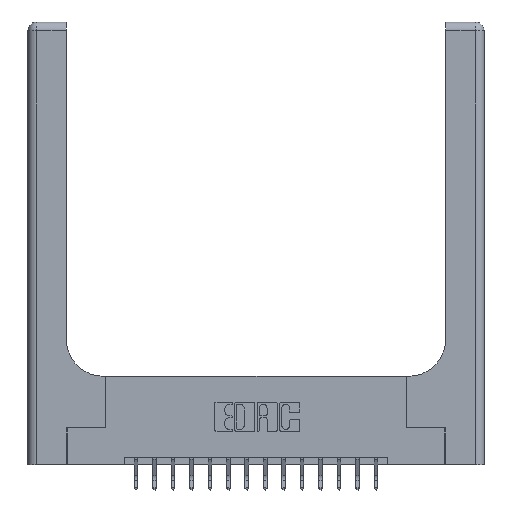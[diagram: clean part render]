
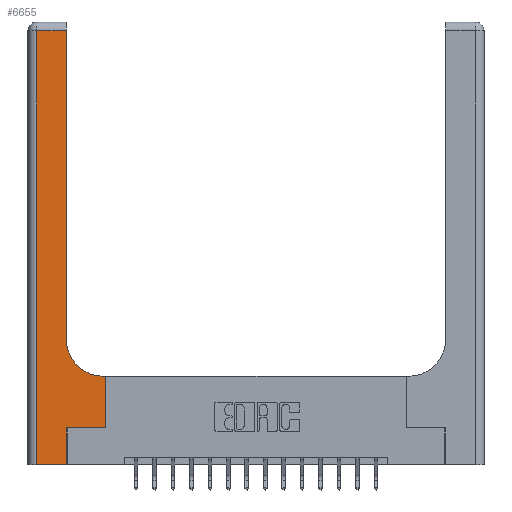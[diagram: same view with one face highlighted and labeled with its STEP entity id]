
A CAD part, top view. The second image highlights one B-rep face of the part: STEP entity #6655.
In plain terms, the highlighted planar face has unit normal (0, 0, 1).
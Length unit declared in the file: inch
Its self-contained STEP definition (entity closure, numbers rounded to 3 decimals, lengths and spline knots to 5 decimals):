
#21 = CARTESIAN_POINT ( 'NONE',  ( 0.265, 0.25, 0.37 ) ) ;
#148 = EDGE_CURVE ( 'NONE', #16364, #14837, #5709, .T. ) ;
#1210 = VECTOR ( 'NONE', #6075, 39.37008 ) ;
#1380 = CARTESIAN_POINT ( 'NONE',  ( 0.265, 0., 0.37 ) ) ;
#1383 = VERTEX_POINT ( 'NONE', #8633 ) ;
#1597 = EDGE_CURVE ( 'NONE', #13291, #3685, #11642, .T. ) ;
#2783 = DIRECTION ( 'NONE',  ( 0., 1., 0. ) ) ;
#3104 = DIRECTION ( 'NONE',  ( 1., 0., 0. ) ) ;
#3341 = DIRECTION ( 'NONE',  ( 0., -1., 0. ) ) ;
#3344 = DIRECTION ( 'NONE',  ( 0., 0., -1. ) ) ;
#3593 = CARTESIAN_POINT ( 'NONE',  ( 0.528, 0.25, 0.37 ) ) ;
#3625 = ORIENTED_EDGE ( 'NONE', *, *, #1597, .T. ) ;
#3685 = VERTEX_POINT ( 'NONE', #4628 ) ;
#3736 = EDGE_CURVE ( 'NONE', #1383, #4712, #17522, .T. ) ;
#4628 = CARTESIAN_POINT ( 'NONE',  ( 0.51, 0.6, 0.37 ) ) ;
#4673 = CARTESIAN_POINT ( 'NONE',  ( 0., 3., 0.37 ) ) ;
#4712 = VERTEX_POINT ( 'NONE', #1380 ) ;
#4831 = LINE ( 'NONE', #5018, #13030 ) ;
#5018 = CARTESIAN_POINT ( 'NONE',  ( 0.26, 3., 0.37 ) ) ;
#5105 = VERTEX_POINT ( 'NONE', #17674 ) ;
#5141 = CARTESIAN_POINT ( 'NONE',  ( 0.528, 0.25, 0.37 ) ) ;
#5709 = LINE ( 'NONE', #21, #10690 ) ;
#5746 = VECTOR ( 'NONE', #2783, 39.37008 ) ;
#5794 = DIRECTION ( 'NONE',  ( 1., 0., 0. ) ) ;
#6075 = DIRECTION ( 'NONE',  ( -1., 0., 0. ) ) ;
#6405 = CARTESIAN_POINT ( 'NONE',  ( 0.51, 0.85, 0.37 ) ) ;
#6655 = ADVANCED_FACE ( 'NONE', ( #17668 ), #13672, .F. ) ;
#6920 = ORIENTED_EDGE ( 'NONE', *, *, #13855, .T. ) ;
#6941 = ORIENTED_EDGE ( 'NONE', *, *, #12118, .T. ) ;
#7020 = EDGE_CURVE ( 'NONE', #5105, #18494, #11986, .T. ) ;
#7134 = EDGE_CURVE ( 'NONE', #7585, #5105, #4831, .T. ) ;
#7201 = ORIENTED_EDGE ( 'NONE', *, *, #7134, .T. ) ;
#7532 = CARTESIAN_POINT ( 'NONE',  ( 0.26, 0.6, 0.37 ) ) ;
#7585 = VERTEX_POINT ( 'NONE', #15391 ) ;
#8453 = EDGE_CURVE ( 'NONE', #4712, #16364, #10010, .T. ) ;
#8633 = CARTESIAN_POINT ( 'NONE',  ( 0.06, 0., 0.37 ) ) ;
#8714 = VECTOR ( 'NONE', #3104, 39.37008 ) ;
#9379 = DIRECTION ( 'NONE',  ( 0., 1., 0. ) ) ;
#10010 = LINE ( 'NONE', #15774, #5746 ) ;
#10304 = EDGE_CURVE ( 'NONE', #18494, #1383, #10725, .T. ) ;
#10545 = DIRECTION ( 'NONE',  ( -1., 0., 0. ) ) ;
#10690 = VECTOR ( 'NONE', #5794, 39.37008 ) ;
#10709 = DIRECTION ( 'NONE',  ( 1., 0., 0. ) ) ;
#10725 = LINE ( 'NONE', #13668, #15811 ) ;
#11341 = VECTOR ( 'NONE', #13161, 39.37008 ) ;
#11504 = AXIS2_PLACEMENT_3D ( 'NONE', #4673, #3344, #10545 ) ;
#11642 = LINE ( 'NONE', #7532, #11341 ) ;
#11924 = ORIENTED_EDGE ( 'NONE', *, *, #7020, .T. ) ;
#11986 = LINE ( 'NONE', #13596, #1210 ) ;
#12118 = EDGE_CURVE ( 'NONE', #3685, #7585, #17019, .T. ) ;
#12216 = DIRECTION ( 'NONE',  ( 0., 1., 0. ) ) ;
#12771 = CARTESIAN_POINT ( 'NONE',  ( 0.528, 0.6, 0.37 ) ) ;
#12981 = ORIENTED_EDGE ( 'NONE', *, *, #10304, .T. ) ;
#12985 = ORIENTED_EDGE ( 'NONE', *, *, #148, .T. ) ;
#13030 = VECTOR ( 'NONE', #12216, 39.37008 ) ;
#13161 = DIRECTION ( 'NONE',  ( -1., 0., 0. ) ) ;
#13291 = VERTEX_POINT ( 'NONE', #12771 ) ;
#13596 = CARTESIAN_POINT ( 'NONE',  ( 0., 2.94, 0.37 ) ) ;
#13668 = CARTESIAN_POINT ( 'NONE',  ( 0.06, 3., 0.37 ) ) ;
#13672 = PLANE ( 'NONE',  #11504 ) ;
#13855 = EDGE_CURVE ( 'NONE', #14837, #13291, #16564, .T. ) ;
#13968 = EDGE_LOOP ( 'NONE', ( #7201, #11924, #12981, #16711, #14301, #12985, #6920, #3625, #6941 ) ) ;
#14301 = ORIENTED_EDGE ( 'NONE', *, *, #8453, .T. ) ;
#14341 = VECTOR ( 'NONE', #9379, 39.37008 ) ;
#14837 = VERTEX_POINT ( 'NONE', #5141 ) ;
#15069 = DIRECTION ( 'NONE',  ( 0., 0., -1. ) ) ;
#15208 = AXIS2_PLACEMENT_3D ( 'NONE', #6405, #15069, #10709 ) ;
#15391 = CARTESIAN_POINT ( 'NONE',  ( 0.26, 0.85, 0.37 ) ) ;
#15774 = CARTESIAN_POINT ( 'NONE',  ( 0.265, 0., 0.37 ) ) ;
#15811 = VECTOR ( 'NONE', #3341, 39.37008 ) ;
#16085 = CARTESIAN_POINT ( 'NONE',  ( 0., 0., 0.37 ) ) ;
#16364 = VERTEX_POINT ( 'NONE', #17866 ) ;
#16564 = LINE ( 'NONE', #3593, #14341 ) ;
#16711 = ORIENTED_EDGE ( 'NONE', *, *, #3736, .T. ) ;
#17019 = CIRCLE ( 'NONE', #15208, 0.25 ) ;
#17522 = LINE ( 'NONE', #16085, #8714 ) ;
#17668 = FACE_OUTER_BOUND ( 'NONE', #13968, .T. ) ;
#17674 = CARTESIAN_POINT ( 'NONE',  ( 0.26, 2.94, 0.37 ) ) ;
#17780 = CARTESIAN_POINT ( 'NONE',  ( 0.06, 2.94, 0.37 ) ) ;
#17866 = CARTESIAN_POINT ( 'NONE',  ( 0.265, 0.25, 0.37 ) ) ;
#18494 = VERTEX_POINT ( 'NONE', #17780 ) ;
